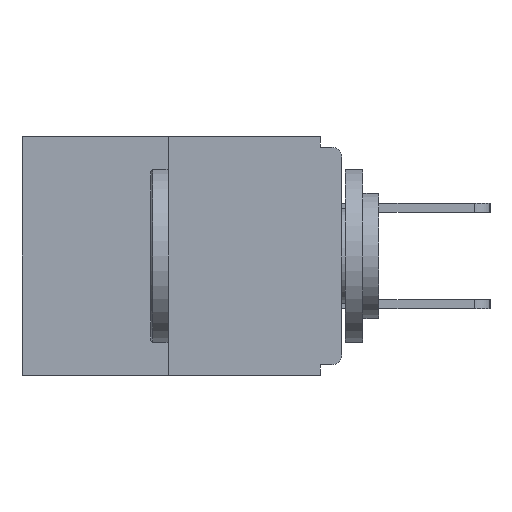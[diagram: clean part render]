
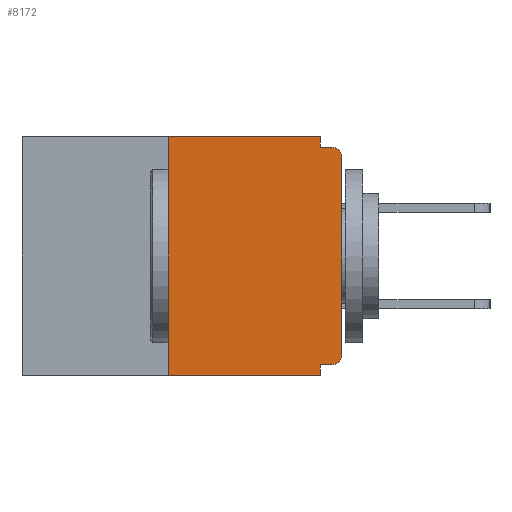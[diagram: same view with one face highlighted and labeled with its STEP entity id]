
A CAD part, left-side view. The second image highlights one B-rep face of the part: STEP entity #8172.
In plain terms, the highlighted planar face has unit normal (-1, 0, 0).
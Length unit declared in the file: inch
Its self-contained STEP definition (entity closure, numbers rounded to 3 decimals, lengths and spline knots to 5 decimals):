
#77 = DIRECTION ( 'NONE',  ( 0., 0., -1. ) ) ;
#472 = DIRECTION ( 'NONE',  ( -1., 0., 0. ) ) ;
#813 = VECTOR ( 'NONE', #9880, 39.37008 ) ;
#1208 = EDGE_CURVE ( 'NONE', #6099, #17841, #22032, .T. ) ;
#1290 = CARTESIAN_POINT ( 'NONE',  ( 0., 0.46, 0. ) ) ;
#1406 = LINE ( 'NONE', #22259, #19267 ) ;
#2543 = CARTESIAN_POINT ( 'NONE',  ( 0., 0.031, -0.343 ) ) ;
#2575 = DIRECTION ( 'NONE',  ( 0., 1., 0. ) ) ;
#2765 = CARTESIAN_POINT ( 'NONE',  ( 0., 0., -0.313 ) ) ;
#2860 = CARTESIAN_POINT ( 'NONE',  ( 0., 0.031, 0. ) ) ;
#2999 = CARTESIAN_POINT ( 'NONE',  ( 0., 0.25, 0. ) ) ;
#3289 = DIRECTION ( 'NONE',  ( 1., 0., 0. ) ) ;
#3559 = AXIS2_PLACEMENT_3D ( 'NONE', #1290, #3289, #18867 ) ;
#3636 = CARTESIAN_POINT ( 'NONE',  ( 0., 0.031, -0.328 ) ) ;
#3842 = ORIENTED_EDGE ( 'NONE', *, *, #1208, .F. ) ;
#4106 = VERTEX_POINT ( 'NONE', #9286 ) ;
#4685 = VECTOR ( 'NONE', #9235, 39.37008 ) ;
#5256 = ORIENTED_EDGE ( 'NONE', *, *, #20044, .F. ) ;
#5279 = AXIS2_PLACEMENT_3D ( 'NONE', #10860, #472, #12207 ) ;
#5355 = ORIENTED_EDGE ( 'NONE', *, *, #21486, .T. ) ;
#5501 = DIRECTION ( 'NONE',  ( 0., 0., 1. ) ) ;
#5772 = CARTESIAN_POINT ( 'NONE',  ( 0., 0.031, 0. ) ) ;
#5889 = CIRCLE ( 'NONE', #5279, 0.015 ) ;
#5985 = DIRECTION ( 'NONE',  ( 0., 0., -1. ) ) ;
#6099 = VERTEX_POINT ( 'NONE', #3636 ) ;
#6171 = EDGE_CURVE ( 'NONE', #20831, #17841, #10523, .T. ) ;
#6224 = ORIENTED_EDGE ( 'NONE', *, *, #6171, .T. ) ;
#6870 = LINE ( 'NONE', #5772, #4685 ) ;
#7213 = ORIENTED_EDGE ( 'NONE', *, *, #16986, .T. ) ;
#7280 = VERTEX_POINT ( 'NONE', #2765 ) ;
#7892 = CARTESIAN_POINT ( 'NONE',  ( 0., 0.031, -0.015 ) ) ;
#8172 = ADVANCED_FACE ( 'NONE', ( #10426 ), #13512, .F. ) ;
#8230 = CARTESIAN_POINT ( 'NONE',  ( 0., 0., -0.03 ) ) ;
#9044 = DIRECTION ( 'NONE',  ( 0., -1., 0. ) ) ;
#9235 = DIRECTION ( 'NONE',  ( 0., 0., -1. ) ) ;
#9286 = CARTESIAN_POINT ( 'NONE',  ( 0., 0.015, -0.328 ) ) ;
#9525 = LINE ( 'NONE', #10281, #10885 ) ;
#9548 = CARTESIAN_POINT ( 'NONE',  ( 0., 0.25, -0.343 ) ) ;
#9880 = DIRECTION ( 'NONE',  ( 0., -1., 0. ) ) ;
#10063 = VERTEX_POINT ( 'NONE', #2860 ) ;
#10119 = ORIENTED_EDGE ( 'NONE', *, *, #16366, .F. ) ;
#10266 = ORIENTED_EDGE ( 'NONE', *, *, #22084, .T. ) ;
#10281 = CARTESIAN_POINT ( 'NONE',  ( 0., 0., -0.015 ) ) ;
#10426 = FACE_OUTER_BOUND ( 'NONE', #21198, .T. ) ;
#10523 = LINE ( 'NONE', #17874, #21590 ) ;
#10615 = CARTESIAN_POINT ( 'NONE',  ( 0., 0.25, 0. ) ) ;
#10860 = CARTESIAN_POINT ( 'NONE',  ( 0., 0.015, -0.313 ) ) ;
#10885 = VECTOR ( 'NONE', #12185, 39.37008 ) ;
#10974 = EDGE_CURVE ( 'NONE', #17712, #11020, #9525, .T. ) ;
#11020 = VERTEX_POINT ( 'NONE', #15430 ) ;
#11834 = LINE ( 'NONE', #10615, #13982 ) ;
#11851 = EDGE_CURVE ( 'NONE', #13926, #10063, #11944, .T. ) ;
#11944 = LINE ( 'NONE', #18410, #813 ) ;
#12185 = DIRECTION ( 'NONE',  ( 0., -1., 0. ) ) ;
#12207 = DIRECTION ( 'NONE',  ( 0., 0., -1. ) ) ;
#12362 = LINE ( 'NONE', #14121, #19894 ) ;
#13352 = DIRECTION ( 'NONE',  ( -1., 0., 0. ) ) ;
#13512 = PLANE ( 'NONE',  #3559 ) ;
#13761 = DIRECTION ( 'NONE',  ( 0., 0., 1. ) ) ;
#13926 = VERTEX_POINT ( 'NONE', #2999 ) ;
#13982 = VECTOR ( 'NONE', #5501, 39.37008 ) ;
#14121 = CARTESIAN_POINT ( 'NONE',  ( 0., 0., -0.328 ) ) ;
#14209 = ORIENTED_EDGE ( 'NONE', *, *, #11851, .F. ) ;
#15430 = CARTESIAN_POINT ( 'NONE',  ( 0., 0.015, -0.015 ) ) ;
#15893 = EDGE_CURVE ( 'NONE', #20831, #13926, #11834, .T. ) ;
#16366 = EDGE_CURVE ( 'NONE', #10063, #17712, #6870, .T. ) ;
#16651 = CIRCLE ( 'NONE', #20885, 0.015 ) ;
#16771 = VERTEX_POINT ( 'NONE', #8230 ) ;
#16986 = EDGE_CURVE ( 'NONE', #7280, #16771, #1406, .T. ) ;
#17455 = VECTOR ( 'NONE', #5985, 39.37008 ) ;
#17668 = ORIENTED_EDGE ( 'NONE', *, *, #10974, .F. ) ;
#17712 = VERTEX_POINT ( 'NONE', #7892 ) ;
#17841 = VERTEX_POINT ( 'NONE', #22023 ) ;
#17874 = CARTESIAN_POINT ( 'NONE',  ( 0., 0.46, -0.343 ) ) ;
#18410 = CARTESIAN_POINT ( 'NONE',  ( 0., 0.46, 0. ) ) ;
#18470 = CARTESIAN_POINT ( 'NONE',  ( 0., 0.015, -0.03 ) ) ;
#18867 = DIRECTION ( 'NONE',  ( 0., 0., -1. ) ) ;
#19267 = VECTOR ( 'NONE', #13761, 39.37008 ) ;
#19359 = ORIENTED_EDGE ( 'NONE', *, *, #15893, .F. ) ;
#19894 = VECTOR ( 'NONE', #2575, 39.37008 ) ;
#20044 = EDGE_CURVE ( 'NONE', #4106, #6099, #12362, .T. ) ;
#20831 = VERTEX_POINT ( 'NONE', #9548 ) ;
#20885 = AXIS2_PLACEMENT_3D ( 'NONE', #18470, #13352, #77 ) ;
#21198 = EDGE_LOOP ( 'NONE', ( #14209, #19359, #6224, #3842, #5256, #10266, #7213, #5355, #17668, #10119 ) ) ;
#21486 = EDGE_CURVE ( 'NONE', #16771, #11020, #16651, .T. ) ;
#21590 = VECTOR ( 'NONE', #9044, 39.37008 ) ;
#22023 = CARTESIAN_POINT ( 'NONE',  ( 0., 0.031, -0.343 ) ) ;
#22032 = LINE ( 'NONE', #2543, #17455 ) ;
#22084 = EDGE_CURVE ( 'NONE', #4106, #7280, #5889, .T. ) ;
#22259 = CARTESIAN_POINT ( 'NONE',  ( 0., 0., 0. ) ) ;
